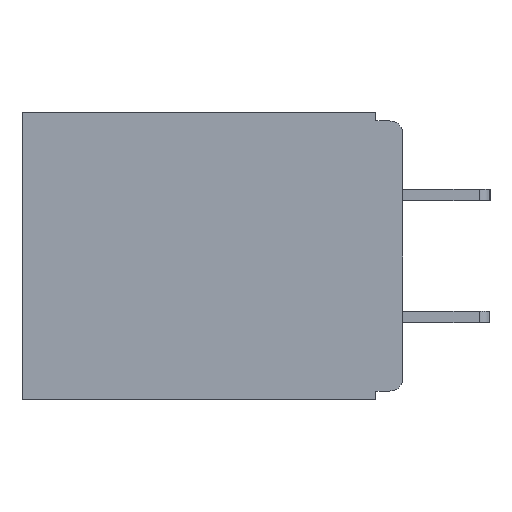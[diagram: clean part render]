
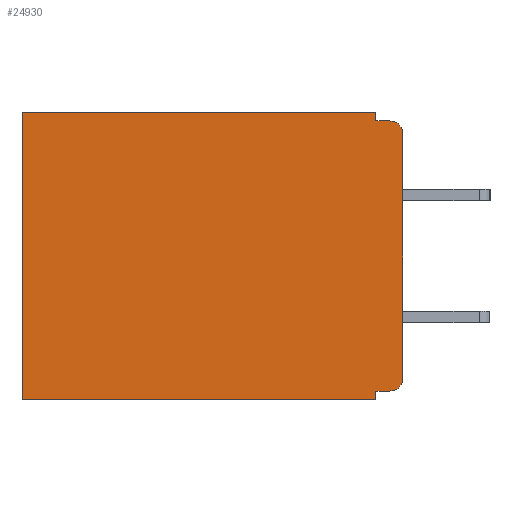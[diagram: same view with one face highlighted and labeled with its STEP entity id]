
A CAD part, left-side view. The second image highlights one B-rep face of the part: STEP entity #24930.
In plain terms, the highlighted planar face has unit normal (-1, 0, 0).
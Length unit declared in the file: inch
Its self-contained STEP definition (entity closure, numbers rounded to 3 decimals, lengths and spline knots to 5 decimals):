
#403 = LINE ( 'NONE', #28986, #5073 ) ;
#413 = VERTEX_POINT ( 'NONE', #8077 ) ;
#466 = DIRECTION ( 'NONE',  ( 0., 0., -1. ) ) ;
#1249 = CARTESIAN_POINT ( 'NONE',  ( 0.3, 0.437, 0. ) ) ;
#1994 = DIRECTION ( 'NONE',  ( 0., 0., -1. ) ) ;
#2187 = DIRECTION ( 'NONE',  ( 0., 1., 0. ) ) ;
#2668 = EDGE_LOOP ( 'NONE', ( #3335, #3006, #4788, #4938, #5273, #6273, #6332, #7019, #6635, #7459 ) ) ;
#2970 = VECTOR ( 'NONE', #26784, 39.37008 ) ;
#3006 = ORIENTED_EDGE ( 'NONE', *, *, #5267, .T. ) ;
#3298 = VERTEX_POINT ( 'NONE', #20781 ) ;
#3335 = ORIENTED_EDGE ( 'NONE', *, *, #25703, .F. ) ;
#3540 = VERTEX_POINT ( 'NONE', #26759 ) ;
#3990 = CARTESIAN_POINT ( 'NONE',  ( 0.3, 0.031, -0.33 ) ) ;
#4057 = FACE_OUTER_BOUND ( 'NONE', #2668, .T. ) ;
#4444 = VECTOR ( 'NONE', #15770, 39.37008 ) ;
#4450 = LINE ( 'NONE', #8154, #9753 ) ;
#4745 = CARTESIAN_POINT ( 'NONE',  ( 0.3, 0., -0.33 ) ) ;
#4788 = ORIENTED_EDGE ( 'NONE', *, *, #16739, .F. ) ;
#4938 = ORIENTED_EDGE ( 'NONE', *, *, #20532, .F. ) ;
#4986 = VECTOR ( 'NONE', #14340, 39.37008 ) ;
#5073 = VECTOR ( 'NONE', #2187, 39.37008 ) ;
#5267 = EDGE_CURVE ( 'NONE', #23989, #3298, #26819, .T. ) ;
#5273 = ORIENTED_EDGE ( 'NONE', *, *, #8248, .T. ) ;
#5437 = VECTOR ( 'NONE', #18300, 39.37008 ) ;
#6121 = CARTESIAN_POINT ( 'NONE',  ( 0.3, 0.015, -0.32 ) ) ;
#6273 = ORIENTED_EDGE ( 'NONE', *, *, #28267, .T. ) ;
#6309 = EDGE_CURVE ( 'NONE', #413, #15823, #4450, .T. ) ;
#6332 = ORIENTED_EDGE ( 'NONE', *, *, #6309, .F. ) ;
#6374 = DIRECTION ( 'NONE',  ( 0., -1., 0. ) ) ;
#6536 = VERTEX_POINT ( 'NONE', #25513 ) ;
#6589 = CARTESIAN_POINT ( 'NONE',  ( 0.3, 0., -0.33 ) ) ;
#6635 = ORIENTED_EDGE ( 'NONE', *, *, #7640, .F. ) ;
#6664 = CIRCLE ( 'NONE', #22475, 0.015 ) ;
#7019 = ORIENTED_EDGE ( 'NONE', *, *, #18987, .F. ) ;
#7459 = ORIENTED_EDGE ( 'NONE', *, *, #23317, .T. ) ;
#7640 = EDGE_CURVE ( 'NONE', #23162, #27691, #403, .T. ) ;
#7966 = DIRECTION ( 'NONE',  ( 0., 1., 0. ) ) ;
#8077 = CARTESIAN_POINT ( 'NONE',  ( 0.3, 0.031, -0.33 ) ) ;
#8154 = CARTESIAN_POINT ( 'NONE',  ( 0.3, 0., -0.33 ) ) ;
#8248 = EDGE_CURVE ( 'NONE', #8836, #14168, #10493, .T. ) ;
#8836 = VERTEX_POINT ( 'NONE', #24343 ) ;
#9753 = VECTOR ( 'NONE', #7966, 39.37008 ) ;
#10493 = LINE ( 'NONE', #28954, #4444 ) ;
#13216 = CARTESIAN_POINT ( 'NONE',  ( 0.3, 0., -0.01 ) ) ;
#13427 = DIRECTION ( 'NONE',  ( 1., 0., 0. ) ) ;
#14112 = DIRECTION ( 'NONE',  ( -1., 0., 0. ) ) ;
#14168 = VERTEX_POINT ( 'NONE', #1249 ) ;
#14340 = DIRECTION ( 'NONE',  ( 0., 0., -1. ) ) ;
#14629 = CARTESIAN_POINT ( 'NONE',  ( 0.3, 0.437, -0.33 ) ) ;
#15342 = LINE ( 'NONE', #3990, #16035 ) ;
#15609 = DIRECTION ( 'NONE',  ( -1., 0., 0. ) ) ;
#15770 = DIRECTION ( 'NONE',  ( 0., 1., 0. ) ) ;
#15803 = AXIS2_PLACEMENT_3D ( 'NONE', #27377, #14112, #466 ) ;
#15823 = VERTEX_POINT ( 'NONE', #14629 ) ;
#16035 = VECTOR ( 'NONE', #17572, 39.37008 ) ;
#16739 = EDGE_CURVE ( 'NONE', #3540, #3298, #26231, .T. ) ;
#17572 = DIRECTION ( 'NONE',  ( 0., 0., -1. ) ) ;
#18300 = DIRECTION ( 'NONE',  ( 0., 0., -1. ) ) ;
#18987 = EDGE_CURVE ( 'NONE', #27691, #413, #15342, .T. ) ;
#19071 = CARTESIAN_POINT ( 'NONE',  ( 0.3, 0., -0.025 ) ) ;
#19137 = AXIS2_PLACEMENT_3D ( 'NONE', #6589, #13427, #28872 ) ;
#20401 = VECTOR ( 'NONE', #6374, 39.37008 ) ;
#20532 = EDGE_CURVE ( 'NONE', #8836, #3540, #28703, .T. ) ;
#20781 = CARTESIAN_POINT ( 'NONE',  ( 0.3, 0.015, -0.01 ) ) ;
#22475 = AXIS2_PLACEMENT_3D ( 'NONE', #28814, #15609, #1994 ) ;
#22498 = CARTESIAN_POINT ( 'NONE',  ( 0.3, 0.437, -0.33 ) ) ;
#23162 = VERTEX_POINT ( 'NONE', #6121 ) ;
#23317 = EDGE_CURVE ( 'NONE', #23162, #6536, #6664, .T. ) ;
#23421 = LINE ( 'NONE', #4745, #5437 ) ;
#23989 = VERTEX_POINT ( 'NONE', #19071 ) ;
#24343 = CARTESIAN_POINT ( 'NONE',  ( 0.3, 0.031, 0. ) ) ;
#24744 = CARTESIAN_POINT ( 'NONE',  ( 0.3, 0.031, -0.32 ) ) ;
#24930 = ADVANCED_FACE ( 'NONE', ( #4057 ), #26739, .F. ) ;
#25513 = CARTESIAN_POINT ( 'NONE',  ( 0.3, 0., -0.305 ) ) ;
#25703 = EDGE_CURVE ( 'NONE', #23989, #6536, #23421, .T. ) ;
#26211 = LINE ( 'NONE', #22498, #2970 ) ;
#26231 = LINE ( 'NONE', #13216, #20401 ) ;
#26739 = PLANE ( 'NONE',  #19137 ) ;
#26759 = CARTESIAN_POINT ( 'NONE',  ( 0.3, 0.031, -0.01 ) ) ;
#26784 = DIRECTION ( 'NONE',  ( 0., 0., -1. ) ) ;
#26819 = CIRCLE ( 'NONE', #15803, 0.015 ) ;
#27377 = CARTESIAN_POINT ( 'NONE',  ( 0.3, 0.015, -0.025 ) ) ;
#27588 = CARTESIAN_POINT ( 'NONE',  ( 0.3, 0.031, 0. ) ) ;
#27691 = VERTEX_POINT ( 'NONE', #24744 ) ;
#28267 = EDGE_CURVE ( 'NONE', #14168, #15823, #26211, .T. ) ;
#28703 = LINE ( 'NONE', #27588, #4986 ) ;
#28814 = CARTESIAN_POINT ( 'NONE',  ( 0.3, 0.015, -0.305 ) ) ;
#28872 = DIRECTION ( 'NONE',  ( 0., 0., -1. ) ) ;
#28954 = CARTESIAN_POINT ( 'NONE',  ( 0.3, 0., 0. ) ) ;
#28986 = CARTESIAN_POINT ( 'NONE',  ( 0.3, 0., -0.32 ) ) ;
